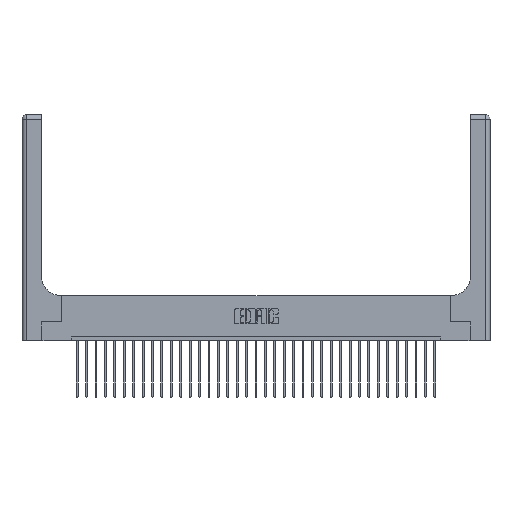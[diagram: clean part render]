
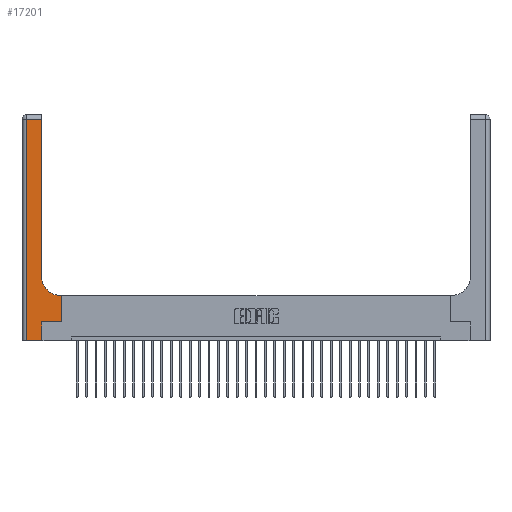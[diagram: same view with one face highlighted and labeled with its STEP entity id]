
A CAD part, top view. The second image highlights one B-rep face of the part: STEP entity #17201.
In plain terms, the highlighted planar face has unit normal (0, 0, 1).
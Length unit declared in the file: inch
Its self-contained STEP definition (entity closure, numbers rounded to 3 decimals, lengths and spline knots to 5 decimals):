
#243 = AXIS2_PLACEMENT_3D ( 'NONE', #22531, #8642, #10957 ) ;
#556 = EDGE_CURVE ( 'NONE', #20278, #19812, #2704, .T. ) ;
#973 = CARTESIAN_POINT ( 'NONE',  ( 0.528, 0.25, 0.37 ) ) ;
#1448 = DIRECTION ( 'NONE',  ( 0., -1., 0. ) ) ;
#1677 = EDGE_CURVE ( 'NONE', #12717, #23663, #26440, .T. ) ;
#2361 = LINE ( 'NONE', #7601, #29733 ) ;
#2386 = CARTESIAN_POINT ( 'NONE',  ( 0.265, 0., 0.37 ) ) ;
#2704 = LINE ( 'NONE', #14620, #5601 ) ;
#2867 = DIRECTION ( 'NONE',  ( -1., 0., 0. ) ) ;
#3172 = EDGE_CURVE ( 'NONE', #23663, #9421, #11592, .T. ) ;
#3272 = VERTEX_POINT ( 'NONE', #973 ) ;
#3900 = ORIENTED_EDGE ( 'NONE', *, *, #13556, .T. ) ;
#4249 = EDGE_LOOP ( 'NONE', ( #17866, #3900, #18450, #5759, #22711, #9209, #12346, #13879, #17733 ) ) ;
#4517 = CARTESIAN_POINT ( 'NONE',  ( 0.26, 2.94, 0.37 ) ) ;
#5095 = EDGE_CURVE ( 'NONE', #11945, #3272, #16138, .T. ) ;
#5477 = VECTOR ( 'NONE', #15133, 39.37008 ) ;
#5601 = VECTOR ( 'NONE', #24093, 39.37008 ) ;
#5759 = ORIENTED_EDGE ( 'NONE', *, *, #3172, .T. ) ;
#5991 = PLANE ( 'NONE',  #15180 ) ;
#6450 = CARTESIAN_POINT ( 'NONE',  ( 0.06, 2.94, 0.37 ) ) ;
#6540 = CARTESIAN_POINT ( 'NONE',  ( 0.265, 0.25, 0.37 ) ) ;
#6546 = CARTESIAN_POINT ( 'NONE',  ( 0.265, 0., 0.37 ) ) ;
#7333 = VECTOR ( 'NONE', #26561, 39.37008 ) ;
#7601 = CARTESIAN_POINT ( 'NONE',  ( 0., 2.94, 0.37 ) ) ;
#8302 = VECTOR ( 'NONE', #9020, 39.37008 ) ;
#8642 = DIRECTION ( 'NONE',  ( 0., 0., -1. ) ) ;
#8782 = CARTESIAN_POINT ( 'NONE',  ( 0., 3., 0.37 ) ) ;
#9020 = DIRECTION ( 'NONE',  ( 0., 1., 0. ) ) ;
#9065 = VECTOR ( 'NONE', #22612, 39.37008 ) ;
#9209 = ORIENTED_EDGE ( 'NONE', *, *, #5095, .T. ) ;
#9421 = VERTEX_POINT ( 'NONE', #2386 ) ;
#10068 = EDGE_CURVE ( 'NONE', #3272, #18471, #22331, .T. ) ;
#10957 = DIRECTION ( 'NONE',  ( 1., 0., 0. ) ) ;
#11592 = LINE ( 'NONE', #28339, #5477 ) ;
#11945 = VERTEX_POINT ( 'NONE', #6540 ) ;
#12346 = ORIENTED_EDGE ( 'NONE', *, *, #10068, .T. ) ;
#12717 = VERTEX_POINT ( 'NONE', #6450 ) ;
#13146 = FACE_OUTER_BOUND ( 'NONE', #4249, .T. ) ;
#13441 = CARTESIAN_POINT ( 'NONE',  ( 0.528, 0.25, 0.37 ) ) ;
#13556 = EDGE_CURVE ( 'NONE', #19812, #12717, #2361, .T. ) ;
#13879 = ORIENTED_EDGE ( 'NONE', *, *, #23386, .T. ) ;
#14620 = CARTESIAN_POINT ( 'NONE',  ( 0.26, 3., 0.37 ) ) ;
#15133 = DIRECTION ( 'NONE',  ( 1., 0., 0. ) ) ;
#15180 = AXIS2_PLACEMENT_3D ( 'NONE', #8782, #15697, #15796 ) ;
#15198 = CARTESIAN_POINT ( 'NONE',  ( 0.06, 3., 0.37 ) ) ;
#15697 = DIRECTION ( 'NONE',  ( 0., 0., -1. ) ) ;
#15761 = VECTOR ( 'NONE', #19426, 39.37008 ) ;
#15796 = DIRECTION ( 'NONE',  ( -1., 0., 0. ) ) ;
#16138 = LINE ( 'NONE', #23820, #15761 ) ;
#17201 = ADVANCED_FACE ( 'NONE', ( #13146 ), #5991, .F. ) ;
#17361 = LINE ( 'NONE', #6546, #9065 ) ;
#17733 = ORIENTED_EDGE ( 'NONE', *, *, #22247, .T. ) ;
#17866 = ORIENTED_EDGE ( 'NONE', *, *, #556, .T. ) ;
#18450 = ORIENTED_EDGE ( 'NONE', *, *, #1677, .T. ) ;
#18471 = VERTEX_POINT ( 'NONE', #25945 ) ;
#19426 = DIRECTION ( 'NONE',  ( 1., 0., 0. ) ) ;
#19538 = VERTEX_POINT ( 'NONE', #23842 ) ;
#19599 = LINE ( 'NONE', #28791, #7333 ) ;
#19812 = VERTEX_POINT ( 'NONE', #4517 ) ;
#20278 = VERTEX_POINT ( 'NONE', #27346 ) ;
#22247 = EDGE_CURVE ( 'NONE', #19538, #20278, #27569, .T. ) ;
#22331 = LINE ( 'NONE', #13441, #8302 ) ;
#22531 = CARTESIAN_POINT ( 'NONE',  ( 0.51, 0.85, 0.37 ) ) ;
#22612 = DIRECTION ( 'NONE',  ( 0., 1., 0. ) ) ;
#22711 = ORIENTED_EDGE ( 'NONE', *, *, #25166, .T. ) ;
#23386 = EDGE_CURVE ( 'NONE', #18471, #19538, #19599, .T. ) ;
#23501 = VECTOR ( 'NONE', #1448, 39.37008 ) ;
#23663 = VERTEX_POINT ( 'NONE', #26519 ) ;
#23820 = CARTESIAN_POINT ( 'NONE',  ( 0.265, 0.25, 0.37 ) ) ;
#23842 = CARTESIAN_POINT ( 'NONE',  ( 0.51, 0.6, 0.37 ) ) ;
#24093 = DIRECTION ( 'NONE',  ( 0., 1., 0. ) ) ;
#25166 = EDGE_CURVE ( 'NONE', #9421, #11945, #17361, .T. ) ;
#25945 = CARTESIAN_POINT ( 'NONE',  ( 0.528, 0.6, 0.37 ) ) ;
#26440 = LINE ( 'NONE', #15198, #23501 ) ;
#26519 = CARTESIAN_POINT ( 'NONE',  ( 0.06, 0., 0.37 ) ) ;
#26561 = DIRECTION ( 'NONE',  ( -1., 0., 0. ) ) ;
#27346 = CARTESIAN_POINT ( 'NONE',  ( 0.26, 0.85, 0.37 ) ) ;
#27569 = CIRCLE ( 'NONE', #243, 0.25 ) ;
#28339 = CARTESIAN_POINT ( 'NONE',  ( 0., 0., 0.37 ) ) ;
#28791 = CARTESIAN_POINT ( 'NONE',  ( 0.26, 0.6, 0.37 ) ) ;
#29733 = VECTOR ( 'NONE', #2867, 39.37008 ) ;
